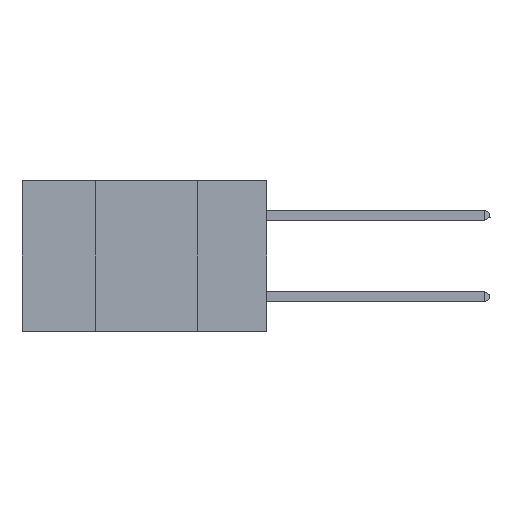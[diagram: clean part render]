
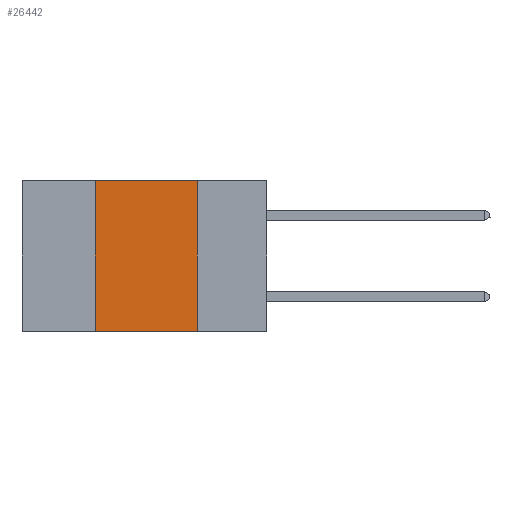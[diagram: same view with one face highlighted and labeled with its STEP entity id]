
A CAD part, left-side view. The second image highlights one B-rep face of the part: STEP entity #26442.
In plain terms, the highlighted planar face has unit normal (-1, 0, 0).
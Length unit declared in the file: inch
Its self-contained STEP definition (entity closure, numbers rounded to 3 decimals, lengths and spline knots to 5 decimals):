
#143 = VERTEX_POINT ( 'NONE', #507 ) ;
#273 = LINE ( 'NONE', #14554, #661 ) ;
#507 = CARTESIAN_POINT ( 'NONE',  ( 0., 0.42, 0. ) ) ;
#615 = CARTESIAN_POINT ( 'NONE',  ( 0., 0.17, 0. ) ) ;
#661 = VECTOR ( 'NONE', #1381, 39.37008 ) ;
#1381 = DIRECTION ( 'NONE',  ( 0., 0., -1. ) ) ;
#1467 = DIRECTION ( 'NONE',  ( 0., 0., -1. ) ) ;
#3671 = PLANE ( 'NONE',  #21349 ) ;
#7072 = VERTEX_POINT ( 'NONE', #19538 ) ;
#7132 = LINE ( 'NONE', #12520, #17507 ) ;
#8262 = DIRECTION ( 'NONE',  ( 1., 0., 0. ) ) ;
#8321 = ORIENTED_EDGE ( 'NONE', *, *, #15521, .F. ) ;
#9087 = ORIENTED_EDGE ( 'NONE', *, *, #21648, .T. ) ;
#9550 = CARTESIAN_POINT ( 'NONE',  ( 0., 0.17, -0.37 ) ) ;
#11547 = DIRECTION ( 'NONE',  ( 0., -1., 0. ) ) ;
#12520 = CARTESIAN_POINT ( 'NONE',  ( 0., 0.42, 0. ) ) ;
#13415 = VERTEX_POINT ( 'NONE', #615 ) ;
#13786 = EDGE_CURVE ( 'NONE', #7072, #143, #7132, .T. ) ;
#14554 = CARTESIAN_POINT ( 'NONE',  ( 0., 0.17, 0. ) ) ;
#15521 = EDGE_CURVE ( 'NONE', #143, #13415, #22043, .T. ) ;
#16422 = EDGE_CURVE ( 'NONE', #13415, #20816, #273, .T. ) ;
#17507 = VECTOR ( 'NONE', #19166, 39.37008 ) ;
#17801 = CARTESIAN_POINT ( 'NONE',  ( 0., 0.6, -0.37 ) ) ;
#18322 = VECTOR ( 'NONE', #11547, 39.37008 ) ;
#19166 = DIRECTION ( 'NONE',  ( 0., 0., 1. ) ) ;
#19538 = CARTESIAN_POINT ( 'NONE',  ( 0., 0.42, -0.37 ) ) ;
#19784 = VECTOR ( 'NONE', #24123, 39.37008 ) ;
#20688 = FACE_OUTER_BOUND ( 'NONE', #22890, .T. ) ;
#20816 = VERTEX_POINT ( 'NONE', #9550 ) ;
#21349 = AXIS2_PLACEMENT_3D ( 'NONE', #25603, #8262, #1467 ) ;
#21648 = EDGE_CURVE ( 'NONE', #7072, #20816, #26946, .T. ) ;
#22043 = LINE ( 'NONE', #24502, #18322 ) ;
#22890 = EDGE_LOOP ( 'NONE', ( #23667, #8321, #26877, #9087 ) ) ;
#23667 = ORIENTED_EDGE ( 'NONE', *, *, #16422, .F. ) ;
#24123 = DIRECTION ( 'NONE',  ( 0., -1., 0. ) ) ;
#24502 = CARTESIAN_POINT ( 'NONE',  ( 0., 0.6, 0. ) ) ;
#25603 = CARTESIAN_POINT ( 'NONE',  ( 0., 0.6, 0. ) ) ;
#26442 = ADVANCED_FACE ( 'NONE', ( #20688 ), #3671, .F. ) ;
#26877 = ORIENTED_EDGE ( 'NONE', *, *, #13786, .F. ) ;
#26946 = LINE ( 'NONE', #17801, #19784 ) ;
